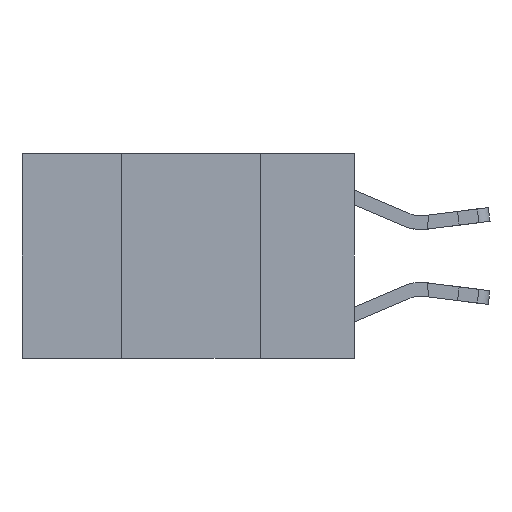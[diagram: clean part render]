
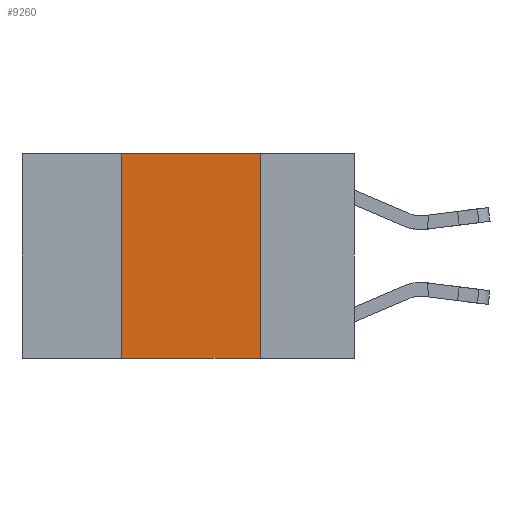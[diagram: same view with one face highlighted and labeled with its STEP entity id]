
A CAD part, left-side view. The second image highlights one B-rep face of the part: STEP entity #9260.
In plain terms, the highlighted planar face has unit normal (-1, 0, 0).
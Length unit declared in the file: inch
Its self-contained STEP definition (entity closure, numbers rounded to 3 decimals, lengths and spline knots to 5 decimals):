
#279 = EDGE_CURVE ( 'NONE', #6017, #9729, #20783, .T. ) ;
#1903 = CARTESIAN_POINT ( 'NONE',  ( 0., 0.42, -0.37 ) ) ;
#3580 = ORIENTED_EDGE ( 'NONE', *, *, #279, .T. ) ;
#3729 = PLANE ( 'NONE',  #9298 ) ;
#4558 = CARTESIAN_POINT ( 'NONE',  ( 0., 0.17, 0. ) ) ;
#4789 = VECTOR ( 'NONE', #10398, 39.37008 ) ;
#5413 = VECTOR ( 'NONE', #15560, 39.37008 ) ;
#6015 = FACE_OUTER_BOUND ( 'NONE', #19307, .T. ) ;
#6017 = VERTEX_POINT ( 'NONE', #1903 ) ;
#6344 = DIRECTION ( 'NONE',  ( 0., 0., -1. ) ) ;
#6658 = VERTEX_POINT ( 'NONE', #20616 ) ;
#6728 = CARTESIAN_POINT ( 'NONE',  ( 0., 0.6, -0.37 ) ) ;
#7086 = ORIENTED_EDGE ( 'NONE', *, *, #18087, .F. ) ;
#8876 = CARTESIAN_POINT ( 'NONE',  ( 0., 0.6, 0. ) ) ;
#9260 = ADVANCED_FACE ( 'NONE', ( #6015 ), #3729, .F. ) ;
#9298 = AXIS2_PLACEMENT_3D ( 'NONE', #8876, #20587, #10600 ) ;
#9729 = VERTEX_POINT ( 'NONE', #13263 ) ;
#9956 = LINE ( 'NONE', #13721, #5413 ) ;
#10058 = DIRECTION ( 'NONE',  ( 0., -1., 0. ) ) ;
#10398 = DIRECTION ( 'NONE',  ( 0., -1., 0. ) ) ;
#10433 = LINE ( 'NONE', #4558, #14324 ) ;
#10600 = DIRECTION ( 'NONE',  ( 0., 0., -1. ) ) ;
#12632 = EDGE_CURVE ( 'NONE', #6017, #21630, #9956, .T. ) ;
#13263 = CARTESIAN_POINT ( 'NONE',  ( 0., 0.17, -0.37 ) ) ;
#13721 = CARTESIAN_POINT ( 'NONE',  ( 0., 0.42, 0. ) ) ;
#13772 = LINE ( 'NONE', #15362, #4789 ) ;
#14324 = VECTOR ( 'NONE', #6344, 39.37008 ) ;
#15362 = CARTESIAN_POINT ( 'NONE',  ( 0., 0.6, 0. ) ) ;
#15560 = DIRECTION ( 'NONE',  ( 0., 0., 1. ) ) ;
#16024 = ORIENTED_EDGE ( 'NONE', *, *, #19028, .F. ) ;
#16541 = ORIENTED_EDGE ( 'NONE', *, *, #12632, .F. ) ;
#18087 = EDGE_CURVE ( 'NONE', #6658, #9729, #10433, .T. ) ;
#19028 = EDGE_CURVE ( 'NONE', #21630, #6658, #13772, .T. ) ;
#19307 = EDGE_LOOP ( 'NONE', ( #7086, #16024, #16541, #3580 ) ) ;
#19586 = CARTESIAN_POINT ( 'NONE',  ( 0., 0.42, 0. ) ) ;
#20250 = VECTOR ( 'NONE', #10058, 39.37008 ) ;
#20587 = DIRECTION ( 'NONE',  ( 1., 0., 0. ) ) ;
#20616 = CARTESIAN_POINT ( 'NONE',  ( 0., 0.17, 0. ) ) ;
#20783 = LINE ( 'NONE', #6728, #20250 ) ;
#21630 = VERTEX_POINT ( 'NONE', #19586 ) ;
